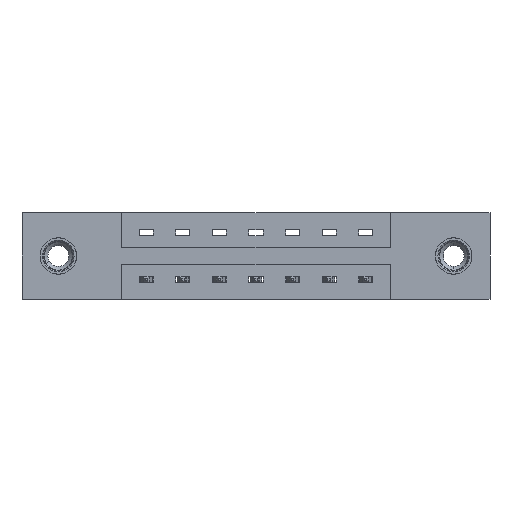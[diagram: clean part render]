
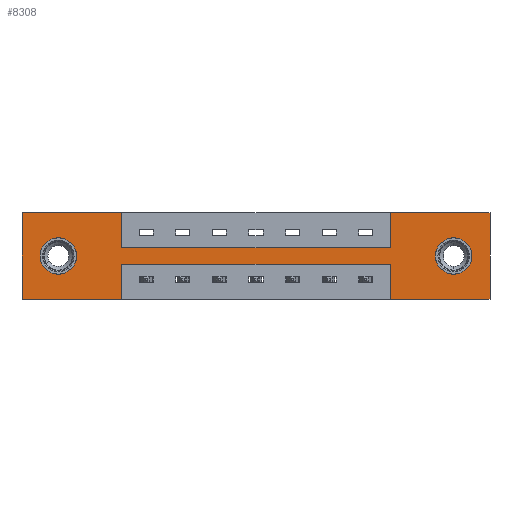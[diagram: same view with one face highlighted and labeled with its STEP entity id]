
A CAD part, front view. The second image highlights one B-rep face of the part: STEP entity #8308.
In plain terms, the highlighted planar face has unit normal (0, -1, 0).
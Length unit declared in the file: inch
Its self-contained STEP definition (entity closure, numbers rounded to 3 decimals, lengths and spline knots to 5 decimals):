
#7 = FACE_OUTER_BOUND ( 'NONE', #561, .T. ) ;
#40 = ORIENTED_EDGE ( 'NONE', *, *, #6434, .F. ) ;
#65 = VERTEX_POINT ( 'NONE', #884 ) ;
#199 = DIRECTION ( 'NONE',  ( 0., 0., 1. ) ) ;
#259 = CIRCLE ( 'NONE', #1076, 0.078 ) ;
#453 = VERTEX_POINT ( 'NONE', #642 ) ;
#561 = EDGE_LOOP ( 'NONE', ( #7230, #4180, #10638, #40, #9392, #1400, #6997, #3060, #1294, #4203, #1912, #7483 ) ) ;
#621 = VERTEX_POINT ( 'NONE', #5894 ) ;
#642 = CARTESIAN_POINT ( 'NONE',  ( 0.155, 0., -0.107 ) ) ;
#662 = PLANE ( 'NONE',  #3485 ) ;
#674 = AXIS2_PLACEMENT_3D ( 'NONE', #5755, #9078, #4012 ) ;
#761 = VECTOR ( 'NONE', #199, 39.37008 ) ;
#778 = CARTESIAN_POINT ( 'NONE',  ( 0.425, 0., -0.15 ) ) ;
#859 = CARTESIAN_POINT ( 'NONE',  ( 1.573, 0., -0.15 ) ) ;
#884 = CARTESIAN_POINT ( 'NONE',  ( 1.843, 0., -0.263 ) ) ;
#915 = EDGE_CURVE ( 'NONE', #5075, #6094, #1778, .T. ) ;
#971 = LINE ( 'NONE', #6026, #8704 ) ;
#994 = LINE ( 'NONE', #2199, #8719 ) ;
#1022 = VERTEX_POINT ( 'NONE', #2137 ) ;
#1076 = AXIS2_PLACEMENT_3D ( 'NONE', #2342, #5688, #7434 ) ;
#1145 = DIRECTION ( 'NONE',  ( 0., 0., -1. ) ) ;
#1153 = CIRCLE ( 'NONE', #674, 0.078 ) ;
#1294 = ORIENTED_EDGE ( 'NONE', *, *, #10179, .F. ) ;
#1400 = ORIENTED_EDGE ( 'NONE', *, *, #5046, .F. ) ;
#1778 = LINE ( 'NONE', #4580, #4068 ) ;
#1825 = DIRECTION ( 'NONE',  ( 0., 1., 0. ) ) ;
#1866 = CARTESIAN_POINT ( 'NONE',  ( 0., 0., 0. ) ) ;
#1912 = ORIENTED_EDGE ( 'NONE', *, *, #915, .F. ) ;
#1949 = CARTESIAN_POINT ( 'NONE',  ( 0.155, 0., -0.263 ) ) ;
#1956 = VERTEX_POINT ( 'NONE', #1949 ) ;
#1963 = EDGE_CURVE ( 'NONE', #3021, #65, #6662, .T. ) ;
#1971 = EDGE_CURVE ( 'NONE', #6094, #1022, #10609, .T. ) ;
#1979 = VERTEX_POINT ( 'NONE', #2162 ) ;
#2057 = CARTESIAN_POINT ( 'NONE',  ( 1.573, 0., -0.37 ) ) ;
#2137 = CARTESIAN_POINT ( 'NONE',  ( 0.425, 0., 0. ) ) ;
#2162 = CARTESIAN_POINT ( 'NONE',  ( 0.425, 0., -0.22 ) ) ;
#2199 = CARTESIAN_POINT ( 'NONE',  ( 0.425, 0., 0. ) ) ;
#2215 = VECTOR ( 'NONE', #3746, 39.37008 ) ;
#2342 = CARTESIAN_POINT ( 'NONE',  ( 0.155, 0., -0.185 ) ) ;
#2505 = LINE ( 'NONE', #7933, #761 ) ;
#2535 = LINE ( 'NONE', #10919, #6093 ) ;
#2796 = FACE_BOUND ( 'NONE', #3749, .T. ) ;
#2971 = EDGE_CURVE ( 'NONE', #1956, #453, #259, .T. ) ;
#3021 = VERTEX_POINT ( 'NONE', #3225 ) ;
#3060 = ORIENTED_EDGE ( 'NONE', *, *, #3436, .F. ) ;
#3102 = VERTEX_POINT ( 'NONE', #859 ) ;
#3225 = CARTESIAN_POINT ( 'NONE',  ( 1.843, 0., -0.107 ) ) ;
#3310 = EDGE_CURVE ( 'NONE', #6637, #8365, #2505, .T. ) ;
#3400 = EDGE_CURVE ( 'NONE', #65, #3021, #1153, .T. ) ;
#3436 = EDGE_CURVE ( 'NONE', #3840, #3102, #8878, .T. ) ;
#3475 = ORIENTED_EDGE ( 'NONE', *, *, #9923, .T. ) ;
#3485 = AXIS2_PLACEMENT_3D ( 'NONE', #7365, #9050, #9901 ) ;
#3506 = CARTESIAN_POINT ( 'NONE',  ( 1.843, 0., -0.185 ) ) ;
#3524 = LINE ( 'NONE', #3873, #6311 ) ;
#3607 = CARTESIAN_POINT ( 'NONE',  ( 0.425, 0., -0.37 ) ) ;
#3624 = DIRECTION ( 'NONE',  ( 0., 0., 1. ) ) ;
#3712 = CARTESIAN_POINT ( 'NONE',  ( 1.998, 0., 0. ) ) ;
#3746 = DIRECTION ( 'NONE',  ( 0., 0., -1. ) ) ;
#3749 = EDGE_LOOP ( 'NONE', ( #8256, #7808 ) ) ;
#3840 = VERTEX_POINT ( 'NONE', #778 ) ;
#3873 = CARTESIAN_POINT ( 'NONE',  ( 1.573, 0., 0. ) ) ;
#4012 = DIRECTION ( 'NONE',  ( 0., 0., -1. ) ) ;
#4068 = VECTOR ( 'NONE', #3624, 39.37008 ) ;
#4180 = ORIENTED_EDGE ( 'NONE', *, *, #5697, .F. ) ;
#4190 = LINE ( 'NONE', #10574, #8051 ) ;
#4203 = ORIENTED_EDGE ( 'NONE', *, *, #1971, .F. ) ;
#4301 = EDGE_CURVE ( 'NONE', #1979, #10129, #6600, .T. ) ;
#4362 = AXIS2_PLACEMENT_3D ( 'NONE', #3506, #1825, #7807 ) ;
#4580 = CARTESIAN_POINT ( 'NONE',  ( 0., 0., 0. ) ) ;
#4622 = CARTESIAN_POINT ( 'NONE',  ( 0., 0., -0.37 ) ) ;
#4654 = EDGE_CURVE ( 'NONE', #3102, #9707, #3524, .T. ) ;
#4775 = FACE_BOUND ( 'NONE', #7615, .T. ) ;
#4838 = DIRECTION ( 'NONE',  ( 0., 1., 0. ) ) ;
#4842 = CARTESIAN_POINT ( 'NONE',  ( 1.573, 0., -0.22 ) ) ;
#4979 = CARTESIAN_POINT ( 'NONE',  ( 1.573, 0., 0. ) ) ;
#5046 = EDGE_CURVE ( 'NONE', #9707, #621, #4190, .T. ) ;
#5075 = VERTEX_POINT ( 'NONE', #9112 ) ;
#5147 = DIRECTION ( 'NONE',  ( 1., 0., 0. ) ) ;
#5371 = CARTESIAN_POINT ( 'NONE',  ( 0.425, 0., -0.37 ) ) ;
#5548 = VECTOR ( 'NONE', #5147, 39.37008 ) ;
#5688 = DIRECTION ( 'NONE',  ( 0., 1., 0. ) ) ;
#5697 = EDGE_CURVE ( 'NONE', #8365, #1979, #971, .T. ) ;
#5737 = DIRECTION ( 'NONE',  ( -1., 0., 0. ) ) ;
#5755 = CARTESIAN_POINT ( 'NONE',  ( 1.843, 0., -0.185 ) ) ;
#5864 = VECTOR ( 'NONE', #6348, 39.37008 ) ;
#5894 = CARTESIAN_POINT ( 'NONE',  ( 1.998, 0., 0. ) ) ;
#6026 = CARTESIAN_POINT ( 'NONE',  ( 0.425, 0., -0.22 ) ) ;
#6093 = VECTOR ( 'NONE', #5737, 39.37008 ) ;
#6094 = VERTEX_POINT ( 'NONE', #1866 ) ;
#6311 = VECTOR ( 'NONE', #9872, 39.37008 ) ;
#6348 = DIRECTION ( 'NONE',  ( 1., 0., 0. ) ) ;
#6382 = DIRECTION ( 'NONE',  ( 0., 0., -1. ) ) ;
#6416 = AXIS2_PLACEMENT_3D ( 'NONE', #9030, #4838, #8451 ) ;
#6434 = EDGE_CURVE ( 'NONE', #8029, #6637, #8954, .T. ) ;
#6466 = ORIENTED_EDGE ( 'NONE', *, *, #2971, .T. ) ;
#6484 = CARTESIAN_POINT ( 'NONE',  ( 0.425, 0., -0.15 ) ) ;
#6600 = LINE ( 'NONE', #5371, #2215 ) ;
#6637 = VERTEX_POINT ( 'NONE', #2057 ) ;
#6662 = CIRCLE ( 'NONE', #4362, 0.078 ) ;
#6821 = DIRECTION ( 'NONE',  ( -1., 0., 0. ) ) ;
#6997 = ORIENTED_EDGE ( 'NONE', *, *, #4654, .F. ) ;
#7230 = ORIENTED_EDGE ( 'NONE', *, *, #4301, .F. ) ;
#7365 = CARTESIAN_POINT ( 'NONE',  ( 0., 0., -0.37 ) ) ;
#7434 = DIRECTION ( 'NONE',  ( 0., 0., 1. ) ) ;
#7457 = EDGE_CURVE ( 'NONE', #621, #8029, #10210, .T. ) ;
#7483 = ORIENTED_EDGE ( 'NONE', *, *, #7941, .F. ) ;
#7615 = EDGE_LOOP ( 'NONE', ( #3475, #6466 ) ) ;
#7807 = DIRECTION ( 'NONE',  ( 0., 0., -1. ) ) ;
#7808 = ORIENTED_EDGE ( 'NONE', *, *, #3400, .T. ) ;
#7933 = CARTESIAN_POINT ( 'NONE',  ( 1.573, 0., -0.37 ) ) ;
#7941 = EDGE_CURVE ( 'NONE', #10129, #5075, #2535, .T. ) ;
#8029 = VERTEX_POINT ( 'NONE', #8478 ) ;
#8051 = VECTOR ( 'NONE', #10659, 39.37008 ) ;
#8256 = ORIENTED_EDGE ( 'NONE', *, *, #1963, .T. ) ;
#8308 = ADVANCED_FACE ( 'NONE', ( #2796, #4775, #7 ), #662, .T. ) ;
#8365 = VERTEX_POINT ( 'NONE', #4842 ) ;
#8451 = DIRECTION ( 'NONE',  ( 0., 0., 1. ) ) ;
#8478 = CARTESIAN_POINT ( 'NONE',  ( 1.998, 0., -0.37 ) ) ;
#8682 = VECTOR ( 'NONE', #9657, 39.37008 ) ;
#8704 = VECTOR ( 'NONE', #6821, 39.37008 ) ;
#8719 = VECTOR ( 'NONE', #6382, 39.37008 ) ;
#8729 = CIRCLE ( 'NONE', #6416, 0.078 ) ;
#8878 = LINE ( 'NONE', #6484, #5548 ) ;
#8954 = LINE ( 'NONE', #4622, #8682 ) ;
#9030 = CARTESIAN_POINT ( 'NONE',  ( 0.155, 0., -0.185 ) ) ;
#9050 = DIRECTION ( 'NONE',  ( 0., -1., 0. ) ) ;
#9078 = DIRECTION ( 'NONE',  ( 0., 1., 0. ) ) ;
#9112 = CARTESIAN_POINT ( 'NONE',  ( 0., 0., -0.37 ) ) ;
#9392 = ORIENTED_EDGE ( 'NONE', *, *, #7457, .F. ) ;
#9412 = VECTOR ( 'NONE', #1145, 39.37008 ) ;
#9657 = DIRECTION ( 'NONE',  ( -1., 0., 0. ) ) ;
#9707 = VERTEX_POINT ( 'NONE', #4979 ) ;
#9872 = DIRECTION ( 'NONE',  ( 0., 0., 1. ) ) ;
#9901 = DIRECTION ( 'NONE',  ( 0., 0., -1. ) ) ;
#9923 = EDGE_CURVE ( 'NONE', #453, #1956, #8729, .T. ) ;
#10129 = VERTEX_POINT ( 'NONE', #3607 ) ;
#10179 = EDGE_CURVE ( 'NONE', #1022, #3840, #994, .T. ) ;
#10210 = LINE ( 'NONE', #3712, #9412 ) ;
#10382 = CARTESIAN_POINT ( 'NONE',  ( 0., 0., 0. ) ) ;
#10574 = CARTESIAN_POINT ( 'NONE',  ( 0., 0., 0. ) ) ;
#10609 = LINE ( 'NONE', #10382, #5864 ) ;
#10638 = ORIENTED_EDGE ( 'NONE', *, *, #3310, .F. ) ;
#10659 = DIRECTION ( 'NONE',  ( 1., 0., 0. ) ) ;
#10919 = CARTESIAN_POINT ( 'NONE',  ( 0., 0., -0.37 ) ) ;
